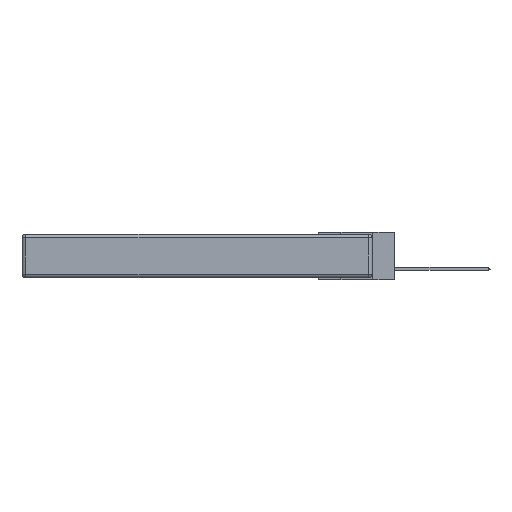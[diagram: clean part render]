
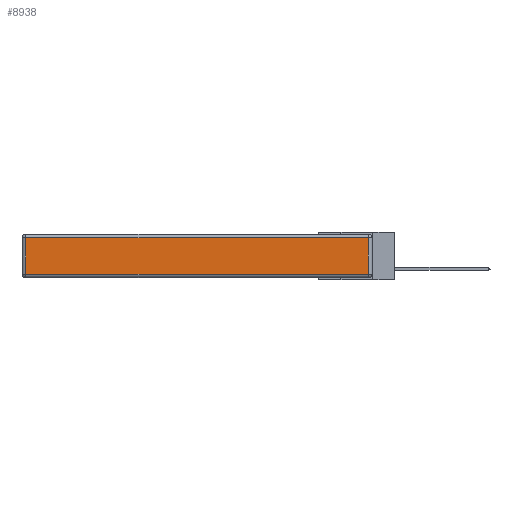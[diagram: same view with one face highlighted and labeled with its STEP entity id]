
A CAD part, left-side view. The second image highlights one B-rep face of the part: STEP entity #8938.
In plain terms, the highlighted planar face has unit normal (-1, 0, 0).
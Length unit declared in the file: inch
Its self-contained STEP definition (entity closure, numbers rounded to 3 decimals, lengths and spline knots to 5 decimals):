
#821 = LINE ( 'NONE', #9799, #7912 ) ;
#1798 = LINE ( 'NONE', #15021, #3550 ) ;
#2898 = CARTESIAN_POINT ( 'NONE',  ( 0., 0., -0.343 ) ) ;
#2932 = CARTESIAN_POINT ( 'NONE',  ( 0., 0.03, -0.343 ) ) ;
#3336 = AXIS2_PLACEMENT_3D ( 'NONE', #2898, #12837, #7889 ) ;
#3550 = VECTOR ( 'NONE', #11071, 39.37008 ) ;
#3756 = LINE ( 'NONE', #2932, #6929 ) ;
#4102 = EDGE_LOOP ( 'NONE', ( #14253, #14059, #6619, #8257 ) ) ;
#4207 = CARTESIAN_POINT ( 'NONE',  ( 0., 0.03, -0.313 ) ) ;
#4666 = VERTEX_POINT ( 'NONE', #11384 ) ;
#5476 = CARTESIAN_POINT ( 'NONE',  ( 0., 0.03, -0.03 ) ) ;
#5496 = CARTESIAN_POINT ( 'NONE',  ( 0., 2.72, -0.03 ) ) ;
#5959 = EDGE_CURVE ( 'NONE', #12673, #6857, #1798, .T. ) ;
#6619 = ORIENTED_EDGE ( 'NONE', *, *, #5959, .T. ) ;
#6857 = VERTEX_POINT ( 'NONE', #5496 ) ;
#6929 = VECTOR ( 'NONE', #13324, 39.37008 ) ;
#7043 = LINE ( 'NONE', #11667, #11297 ) ;
#7610 = VERTEX_POINT ( 'NONE', #4207 ) ;
#7889 = DIRECTION ( 'NONE',  ( 0., 0., 1. ) ) ;
#7912 = VECTOR ( 'NONE', #14796, 39.37008 ) ;
#8257 = ORIENTED_EDGE ( 'NONE', *, *, #8413, .T. ) ;
#8413 = EDGE_CURVE ( 'NONE', #6857, #4666, #7043, .T. ) ;
#8938 = ADVANCED_FACE ( 'NONE', ( #12475 ), #11577, .T. ) ;
#9799 = CARTESIAN_POINT ( 'NONE',  ( 0., 0., -0.313 ) ) ;
#10570 = EDGE_CURVE ( 'NONE', #4666, #7610, #821, .T. ) ;
#11058 = EDGE_CURVE ( 'NONE', #7610, #12673, #3756, .T. ) ;
#11071 = DIRECTION ( 'NONE',  ( 0., 1., 0. ) ) ;
#11297 = VECTOR ( 'NONE', #15431, 39.37008 ) ;
#11384 = CARTESIAN_POINT ( 'NONE',  ( 0., 2.72, -0.313 ) ) ;
#11577 = PLANE ( 'NONE',  #3336 ) ;
#11667 = CARTESIAN_POINT ( 'NONE',  ( 0., 2.72, -0.343 ) ) ;
#12475 = FACE_OUTER_BOUND ( 'NONE', #4102, .T. ) ;
#12673 = VERTEX_POINT ( 'NONE', #5476 ) ;
#12837 = DIRECTION ( 'NONE',  ( -1., 0., 0. ) ) ;
#13324 = DIRECTION ( 'NONE',  ( 0., 0., 1. ) ) ;
#14059 = ORIENTED_EDGE ( 'NONE', *, *, #11058, .T. ) ;
#14253 = ORIENTED_EDGE ( 'NONE', *, *, #10570, .T. ) ;
#14796 = DIRECTION ( 'NONE',  ( 0., -1., 0. ) ) ;
#15021 = CARTESIAN_POINT ( 'NONE',  ( 0., 2.75, -0.03 ) ) ;
#15431 = DIRECTION ( 'NONE',  ( 0., 0., -1. ) ) ;
